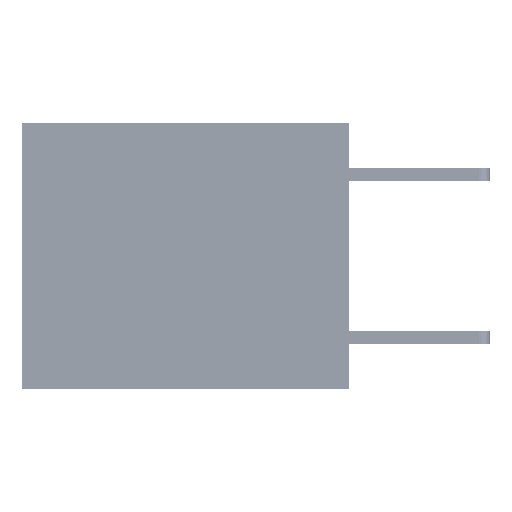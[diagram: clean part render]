
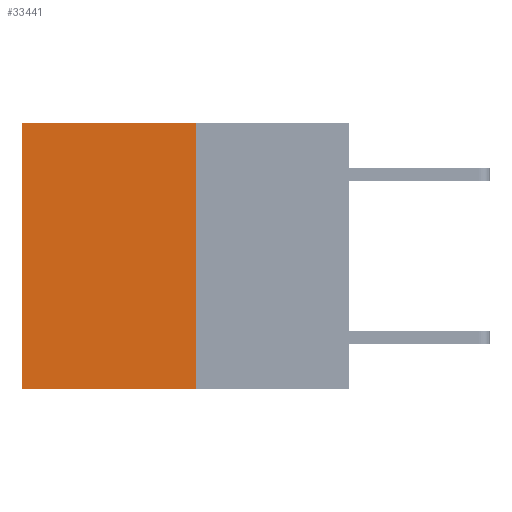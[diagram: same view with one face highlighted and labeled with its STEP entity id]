
A CAD part, left-side view. The second image highlights one B-rep face of the part: STEP entity #33441.
In plain terms, the highlighted planar face has unit normal (-1, 0, 0).
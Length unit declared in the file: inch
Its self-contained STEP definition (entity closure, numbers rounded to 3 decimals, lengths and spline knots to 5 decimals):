
#353 = VECTOR ( 'NONE', #9316, 39.37008 ) ;
#728 = LINE ( 'NONE', #13059, #21229 ) ;
#1466 = CARTESIAN_POINT ( 'NONE',  ( 0.3165, 0.6, -0.49 ) ) ;
#1579 = AXIS2_PLACEMENT_3D ( 'NONE', #3465, #24559, #3135 ) ;
#1867 = LINE ( 'NONE', #15058, #30388 ) ;
#2650 = EDGE_CURVE ( 'NONE', #6840, #21253, #12625, .T. ) ;
#3135 = DIRECTION ( 'NONE',  ( 0., 0., -1. ) ) ;
#3465 = CARTESIAN_POINT ( 'NONE',  ( 0.3165, 0.28, -0.49 ) ) ;
#4958 = DIRECTION ( 'NONE',  ( 0., 0., -1. ) ) ;
#6630 = CARTESIAN_POINT ( 'NONE',  ( 0.3165, 0.28, -0.49 ) ) ;
#6840 = VERTEX_POINT ( 'NONE', #14146 ) ;
#9316 = DIRECTION ( 'NONE',  ( 0., 1., 0. ) ) ;
#11199 = VERTEX_POINT ( 'NONE', #29190 ) ;
#12625 = LINE ( 'NONE', #30715, #26828 ) ;
#13059 = CARTESIAN_POINT ( 'NONE',  ( 0.3165, 0.28, -0.49 ) ) ;
#13558 = CARTESIAN_POINT ( 'NONE',  ( 0.3165, 0.6, 0. ) ) ;
#14146 = CARTESIAN_POINT ( 'NONE',  ( 0.3165, 0.28, 0. ) ) ;
#14795 = ORIENTED_EDGE ( 'NONE', *, *, #30015, .F. ) ;
#15058 = CARTESIAN_POINT ( 'NONE',  ( 0.3165, 0.6, -0.49 ) ) ;
#15687 = EDGE_CURVE ( 'NONE', #6840, #11199, #728, .T. ) ;
#16252 = ORIENTED_EDGE ( 'NONE', *, *, #2650, .T. ) ;
#17586 = FACE_OUTER_BOUND ( 'NONE', #31159, .T. ) ;
#18373 = ORIENTED_EDGE ( 'NONE', *, *, #15687, .F. ) ;
#19200 = PLANE ( 'NONE',  #1579 ) ;
#21229 = VECTOR ( 'NONE', #4958, 39.37008 ) ;
#21253 = VERTEX_POINT ( 'NONE', #13558 ) ;
#21977 = EDGE_CURVE ( 'NONE', #21253, #25821, #1867, .T. ) ;
#23796 = LINE ( 'NONE', #6630, #353 ) ;
#24559 = DIRECTION ( 'NONE',  ( 1., 0., 0. ) ) ;
#25821 = VERTEX_POINT ( 'NONE', #1466 ) ;
#26075 = ORIENTED_EDGE ( 'NONE', *, *, #21977, .T. ) ;
#26828 = VECTOR ( 'NONE', #33398, 39.37008 ) ;
#28757 = DIRECTION ( 'NONE',  ( 0., 0., -1. ) ) ;
#29190 = CARTESIAN_POINT ( 'NONE',  ( 0.3165, 0.28, -0.49 ) ) ;
#30015 = EDGE_CURVE ( 'NONE', #11199, #25821, #23796, .T. ) ;
#30388 = VECTOR ( 'NONE', #28757, 39.37008 ) ;
#30715 = CARTESIAN_POINT ( 'NONE',  ( 0.3165, 0.28, 0. ) ) ;
#31159 = EDGE_LOOP ( 'NONE', ( #26075, #14795, #18373, #16252 ) ) ;
#33398 = DIRECTION ( 'NONE',  ( 0., 1., 0. ) ) ;
#33441 = ADVANCED_FACE ( 'NONE', ( #17586 ), #19200, .F. ) ;
